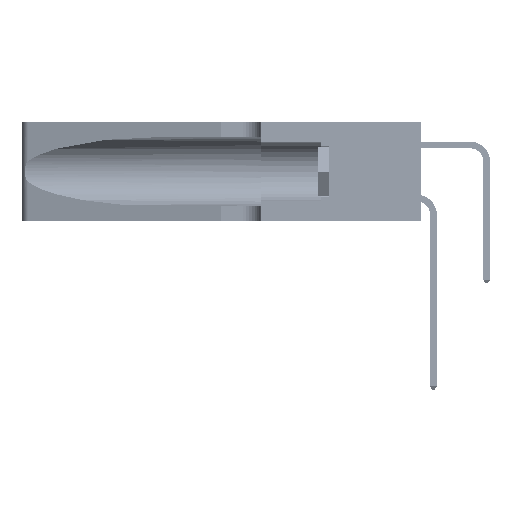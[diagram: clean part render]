
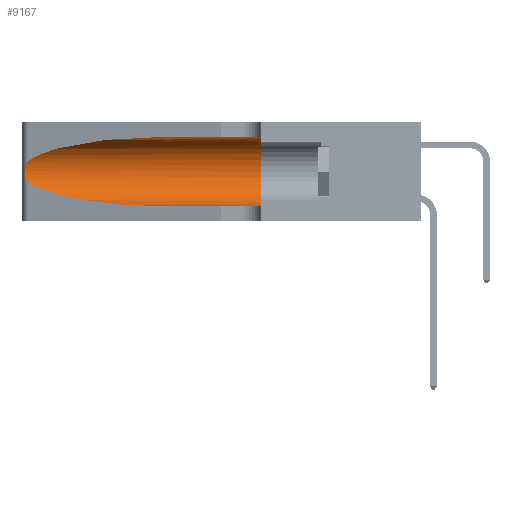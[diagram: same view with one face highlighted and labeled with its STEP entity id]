
A CAD part, left-side view. The second image highlights one B-rep face of the part: STEP entity #9167.
In plain terms, the highlighted cylindrical face has radius 3.308 mm (diameter 6.617 mm), a partial arc.
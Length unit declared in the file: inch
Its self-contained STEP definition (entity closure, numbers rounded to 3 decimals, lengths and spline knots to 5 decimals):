
#1322 = EDGE_CURVE ( 'NONE', #13788, #32182, #21617, .T. ) ;
#1650 = CARTESIAN_POINT ( 'NONE',  ( 0.25487, 1.22718, 0.14631 ) ) ;
#2014 = CARTESIAN_POINT ( 'NONE',  ( 0.25487, 1.22718, 0.14631 ) ) ;
#2500 = CARTESIAN_POINT ( 'NONE',  ( 0.25856, 1.23593, 0.16098 ) ) ;
#2781 = CARTESIAN_POINT ( 'NONE',  ( 0.1305, 1.61858, 0.05475 ) ) ;
#3021 = ORIENTED_EDGE ( 'NONE', *, *, #12272, .T. ) ;
#4162 = CARTESIAN_POINT ( 'NONE',  ( 0.1305, 1.61858, 0.185 ) ) ;
#4510 = CARTESIAN_POINT ( 'NONE',  ( 0.2373, 1.15595, 0.28018 ) ) ;
#6218 = CARTESIAN_POINT ( 'NONE',  ( 0.25639, 1.23184, 0.21858 ) ) ;
#6625 = EDGE_CURVE ( 'NONE', #32369, #28057, #47656, .T. ) ;
#6823 =( BOUNDED_CURVE ( )  B_SPLINE_CURVE ( 3, ( #11450, #22915, #4510, #37692 ),
 .UNSPECIFIED., .F., .F. ) 
 B_SPLINE_CURVE_WITH_KNOTS ( ( 4, 4 ),
 ( 1.5708, 2.84003 ),
 .UNSPECIFIED. ) 
 CURVE ( )  GEOMETRIC_REPRESENTATION_ITEM ( )  RATIONAL_B_SPLINE_CURVE ( ( 1., 0.87, 0.87, 1. ) ) 
 REPRESENTATION_ITEM ( '' )  );
#9167 = ADVANCED_FACE ( 'NONE', ( #28499 ), #9453, .F. ) ;
#9453 = CYLINDRICAL_SURFACE ( 'NONE', #46927, 0.13025 ) ;
#9752 = CARTESIAN_POINT ( 'NONE',  ( 0.1305, 0.72297, 0.05475 ) ) ;
#10567 = CARTESIAN_POINT ( 'NONE',  ( 0.25555, 1.22993, 0.14849 ) ) ;
#11450 = CARTESIAN_POINT ( 'NONE',  ( 0.1305, 0.72297, 0.31525 ) ) ;
#12272 = EDGE_CURVE ( 'NONE', #35419, #13788, #6823, .T. ) ;
#13107 = CARTESIAN_POINT ( 'NONE',  ( 0.1305, 0.72297, 0.05475 ) ) ;
#13187 = EDGE_CURVE ( 'NONE', #35419, #32369, #43668, .T. ) ;
#13499 = CARTESIAN_POINT ( 'NONE',  ( 0.26075, 1.23896, 0.19203 ) ) ;
#13788 = VERTEX_POINT ( 'NONE', #34739 ) ;
#14090 = DIRECTION ( 'NONE',  ( 0., -1., 0. ) ) ;
#15098 = CARTESIAN_POINT ( 'NONE',  ( 0.25487, 1.22718, 0.14631 ) ) ;
#15405 =( BOUNDED_CURVE ( )  B_SPLINE_CURVE ( 3, ( #2014, #31831, #38917, #9752 ),
 .UNSPECIFIED., .F., .F. ) 
 B_SPLINE_CURVE_WITH_KNOTS ( ( 4, 4 ),
 ( 3.44316, 4.71239 ),
 .UNSPECIFIED. ) 
 CURVE ( )  GEOMETRIC_REPRESENTATION_ITEM ( )  RATIONAL_B_SPLINE_CURVE ( ( 1., 0.87, 0.87, 1. ) ) 
 REPRESENTATION_ITEM ( '' )  );
#16423 = DIRECTION ( 'NONE',  ( 0., -1., 0. ) ) ;
#16734 = ORIENTED_EDGE ( 'NONE', *, *, #40105, .T. ) ;
#21234 = VECTOR ( 'NONE', #16423, 39.37008 ) ;
#21521 = ORIENTED_EDGE ( 'NONE', *, *, #1322, .T. ) ;
#21617 = B_SPLINE_CURVE_WITH_KNOTS ( 'NONE', 3,
 ( #24946, #42796, #6218, #24458, #31846, #25111, #13499, #46688, #24626, #2500, #26407, #22846, #10567, #15098 ),
 .UNSPECIFIED., .F., .F.,
 ( 4, 2, 2, 2, 2, 2, 4 ),
 ( 0., 0.00027, 0.00053, 0.00107, 0.0016, 0.00187, 0.00214 ),
 .UNSPECIFIED. ) ;
#22449 = CARTESIAN_POINT ( 'NONE',  ( 0.1305, 0.35, 0.05475 ) ) ;
#22846 = CARTESIAN_POINT ( 'NONE',  ( 0.25639, 1.23186, 0.15144 ) ) ;
#22915 = CARTESIAN_POINT ( 'NONE',  ( 0.18966, 0.96281, 0.31525 ) ) ;
#24071 = DIRECTION ( 'NONE',  ( 0., 1., 0. ) ) ;
#24381 = DIRECTION ( 'NONE',  ( 0., 0., 1. ) ) ;
#24458 = CARTESIAN_POINT ( 'NONE',  ( 0.25787, 1.23484, 0.2124 ) ) ;
#24626 = CARTESIAN_POINT ( 'NONE',  ( 0.26017, 1.23833, 0.17102 ) ) ;
#24946 = CARTESIAN_POINT ( 'NONE',  ( 0.25487, 1.22718, 0.22369 ) ) ;
#25111 = CARTESIAN_POINT ( 'NONE',  ( 0.26018, 1.23835, 0.19895 ) ) ;
#25281 = AXIS2_PLACEMENT_3D ( 'NONE', #43051, #24071, #24381 ) ;
#25795 = VERTEX_POINT ( 'NONE', #13107 ) ;
#26407 = CARTESIAN_POINT ( 'NONE',  ( 0.25789, 1.23486, 0.15765 ) ) ;
#27700 = CARTESIAN_POINT ( 'NONE',  ( 0.1305, 1.61858, 0.31525 ) ) ;
#28057 = VERTEX_POINT ( 'NONE', #22449 ) ;
#28499 = FACE_OUTER_BOUND ( 'NONE', #47419, .T. ) ;
#30130 = LINE ( 'NONE', #2781, #32435 ) ;
#30261 = EDGE_CURVE ( 'NONE', #32182, #25795, #15405, .T. ) ;
#31831 = CARTESIAN_POINT ( 'NONE',  ( 0.2373, 1.15595, 0.08982 ) ) ;
#31846 = CARTESIAN_POINT ( 'NONE',  ( 0.25854, 1.2359, 0.20912 ) ) ;
#32182 = VERTEX_POINT ( 'NONE', #1650 ) ;
#32369 = VERTEX_POINT ( 'NONE', #42586 ) ;
#32435 = VECTOR ( 'NONE', #14090, 39.37008 ) ;
#34013 = DIRECTION ( 'NONE',  ( 0., 0., -1. ) ) ;
#34739 = CARTESIAN_POINT ( 'NONE',  ( 0.25487, 1.22718, 0.22369 ) ) ;
#35360 = ORIENTED_EDGE ( 'NONE', *, *, #13187, .F. ) ;
#35419 = VERTEX_POINT ( 'NONE', #38318 ) ;
#37527 = DIRECTION ( 'NONE',  ( 0., -1., 0. ) ) ;
#37692 = CARTESIAN_POINT ( 'NONE',  ( 0.25487, 1.22718, 0.22369 ) ) ;
#38318 = CARTESIAN_POINT ( 'NONE',  ( 0.1305, 0.72297, 0.31525 ) ) ;
#38917 = CARTESIAN_POINT ( 'NONE',  ( 0.18966, 0.96281, 0.05475 ) ) ;
#40105 = EDGE_CURVE ( 'NONE', #25795, #28057, #30130, .T. ) ;
#40878 = ORIENTED_EDGE ( 'NONE', *, *, #30261, .T. ) ;
#42586 = CARTESIAN_POINT ( 'NONE',  ( 0.1305, 0.35, 0.31525 ) ) ;
#42796 = CARTESIAN_POINT ( 'NONE',  ( 0.25555, 1.22994, 0.2215 ) ) ;
#43051 = CARTESIAN_POINT ( 'NONE',  ( 0.1305, 0.35, 0.185 ) ) ;
#43668 = LINE ( 'NONE', #27700, #21234 ) ;
#45966 = ORIENTED_EDGE ( 'NONE', *, *, #6625, .F. ) ;
#46688 = CARTESIAN_POINT ( 'NONE',  ( 0.26075, 1.23896, 0.178 ) ) ;
#46927 = AXIS2_PLACEMENT_3D ( 'NONE', #4162, #37527, #34013 ) ;
#47419 = EDGE_LOOP ( 'NONE', ( #3021, #21521, #40878, #16734, #45966, #35360 ) ) ;
#47656 = CIRCLE ( 'NONE', #25281, 0.13025 ) ;
